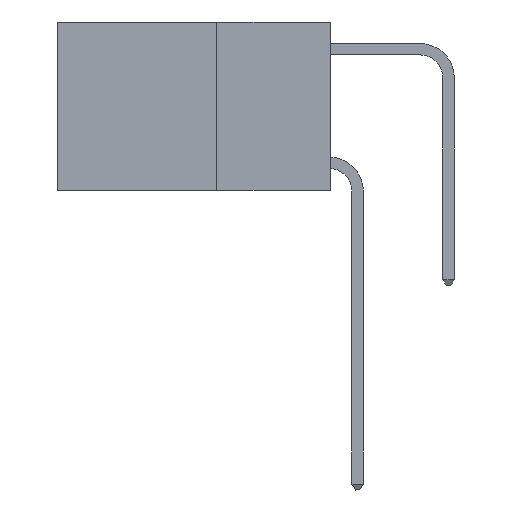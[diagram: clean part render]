
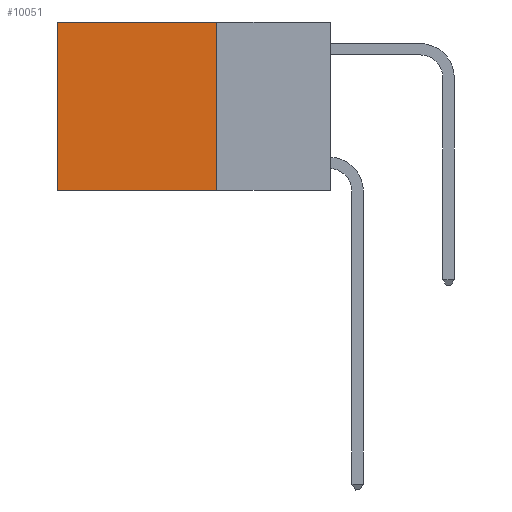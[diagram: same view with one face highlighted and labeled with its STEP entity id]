
A CAD part, left-side view. The second image highlights one B-rep face of the part: STEP entity #10051.
In plain terms, the highlighted planar face has unit normal (-1, 0, 0).
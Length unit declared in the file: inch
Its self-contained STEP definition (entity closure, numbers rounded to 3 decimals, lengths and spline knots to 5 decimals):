
#282 = VECTOR ( 'NONE', #13678, 39.37008 ) ;
#757 = VERTEX_POINT ( 'NONE', #21038 ) ;
#966 = DIRECTION ( 'NONE',  ( 0., 0., -1. ) ) ;
#1532 = CARTESIAN_POINT ( 'NONE',  ( 0.2625, 0.25, -0.37 ) ) ;
#4374 = CARTESIAN_POINT ( 'NONE',  ( 0.2625, 0.25, 0. ) ) ;
#5472 = LINE ( 'NONE', #1532, #14285 ) ;
#5678 = CARTESIAN_POINT ( 'NONE',  ( 0.2625, 0.6, -0.37 ) ) ;
#6510 = LINE ( 'NONE', #10053, #282 ) ;
#7169 = VERTEX_POINT ( 'NONE', #8338 ) ;
#7175 = AXIS2_PLACEMENT_3D ( 'NONE', #4374, #20544, #17126 ) ;
#8338 = CARTESIAN_POINT ( 'NONE',  ( 0.2625, 0.6, 0. ) ) ;
#9065 = CARTESIAN_POINT ( 'NONE',  ( 0.2625, 0.25, 0. ) ) ;
#9396 = ORIENTED_EDGE ( 'NONE', *, *, #12835, .T. ) ;
#10051 = ADVANCED_FACE ( 'NONE', ( #20418 ), #13372, .F. ) ;
#10053 = CARTESIAN_POINT ( 'NONE',  ( 0.2625, 0.25, 0. ) ) ;
#10858 = VERTEX_POINT ( 'NONE', #5678 ) ;
#11582 = LINE ( 'NONE', #11691, #12638 ) ;
#11691 = CARTESIAN_POINT ( 'NONE',  ( 0.2625, 0.6, 0. ) ) ;
#11900 = ORIENTED_EDGE ( 'NONE', *, *, #20256, .F. ) ;
#12083 = VECTOR ( 'NONE', #22237, 39.37008 ) ;
#12638 = VECTOR ( 'NONE', #966, 39.37008 ) ;
#12835 = EDGE_CURVE ( 'NONE', #15185, #7169, #20686, .T. ) ;
#13372 = PLANE ( 'NONE',  #7175 ) ;
#13678 = DIRECTION ( 'NONE',  ( 0., 0., -1. ) ) ;
#14253 = DIRECTION ( 'NONE',  ( 0., 1., 0. ) ) ;
#14285 = VECTOR ( 'NONE', #14253, 39.37008 ) ;
#15031 = CARTESIAN_POINT ( 'NONE',  ( 0.2625, 0.25, 0. ) ) ;
#15185 = VERTEX_POINT ( 'NONE', #9065 ) ;
#16130 = ORIENTED_EDGE ( 'NONE', *, *, #21420, .T. ) ;
#16502 = EDGE_CURVE ( 'NONE', #757, #10858, #5472, .T. ) ;
#17126 = DIRECTION ( 'NONE',  ( 0., 0., -1. ) ) ;
#18048 = EDGE_LOOP ( 'NONE', ( #16130, #20568, #11900, #9396 ) ) ;
#20256 = EDGE_CURVE ( 'NONE', #15185, #757, #6510, .T. ) ;
#20418 = FACE_OUTER_BOUND ( 'NONE', #18048, .T. ) ;
#20544 = DIRECTION ( 'NONE',  ( 1., 0., 0. ) ) ;
#20568 = ORIENTED_EDGE ( 'NONE', *, *, #16502, .F. ) ;
#20686 = LINE ( 'NONE', #15031, #12083 ) ;
#21038 = CARTESIAN_POINT ( 'NONE',  ( 0.2625, 0.25, -0.37 ) ) ;
#21420 = EDGE_CURVE ( 'NONE', #7169, #10858, #11582, .T. ) ;
#22237 = DIRECTION ( 'NONE',  ( 0., 1., 0. ) ) ;
